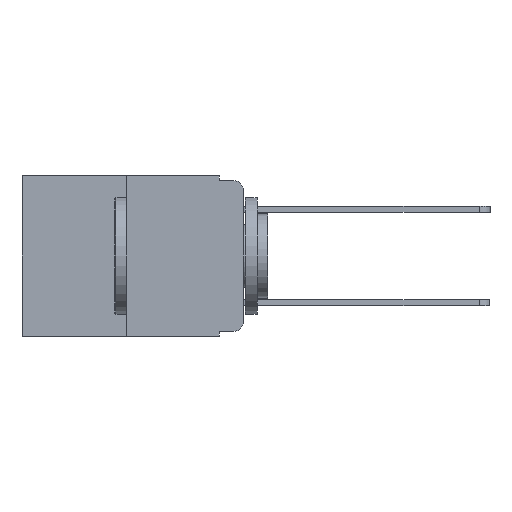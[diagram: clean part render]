
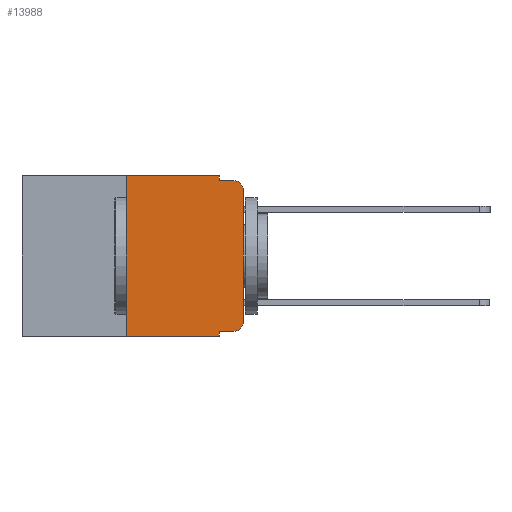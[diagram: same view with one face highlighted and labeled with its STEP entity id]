
A CAD part, left-side view. The second image highlights one B-rep face of the part: STEP entity #13988.
In plain terms, the highlighted planar face has unit normal (-1, 0, 0).
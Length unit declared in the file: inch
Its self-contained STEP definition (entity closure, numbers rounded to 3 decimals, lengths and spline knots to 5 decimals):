
#233 = EDGE_CURVE ( 'NONE', #7229, #4358, #17856, .T. ) ;
#365 = DIRECTION ( 'NONE',  ( 0., 0., 1. ) ) ;
#557 = LINE ( 'NONE', #856, #15821 ) ;
#856 = CARTESIAN_POINT ( 'NONE',  ( 0., 0.051, -0.01 ) ) ;
#885 = VECTOR ( 'NONE', #15459, 39.37008 ) ;
#1160 = VECTOR ( 'NONE', #2512, 39.37008 ) ;
#1750 = CARTESIAN_POINT ( 'NONE',  ( 0., 0.25, -0.343 ) ) ;
#2093 = ORIENTED_EDGE ( 'NONE', *, *, #9291, .F. ) ;
#2106 = ORIENTED_EDGE ( 'NONE', *, *, #10698, .F. ) ;
#2223 = CARTESIAN_POINT ( 'NONE',  ( 0., 0.02, -0.333 ) ) ;
#2512 = DIRECTION ( 'NONE',  ( 0., 0., 1. ) ) ;
#2616 = VERTEX_POINT ( 'NONE', #1750 ) ;
#2858 = ORIENTED_EDGE ( 'NONE', *, *, #9841, .T. ) ;
#3598 = LINE ( 'NONE', #12702, #11689 ) ;
#3950 = PLANE ( 'NONE',  #15090 ) ;
#4358 = VERTEX_POINT ( 'NONE', #13823 ) ;
#4474 = LINE ( 'NONE', #4968, #10679 ) ;
#4842 = ORIENTED_EDGE ( 'NONE', *, *, #16781, .T. ) ;
#4890 = CARTESIAN_POINT ( 'NONE',  ( 0., 0.051, 0. ) ) ;
#4935 = EDGE_LOOP ( 'NONE', ( #10047, #17041, #8863, #15759, #2093, #6054, #4842, #2106, #17639, #2858 ) ) ;
#4968 = CARTESIAN_POINT ( 'NONE',  ( 0., 0.473, 0. ) ) ;
#5125 = CARTESIAN_POINT ( 'NONE',  ( 0., 0.051, 0. ) ) ;
#5420 = LINE ( 'NONE', #16040, #1160 ) ;
#5471 = CARTESIAN_POINT ( 'NONE',  ( 0., 0.473, 0. ) ) ;
#5538 = DIRECTION ( 'NONE',  ( 0., 0., -1. ) ) ;
#5848 = DIRECTION ( 'NONE',  ( 0., -1., 0. ) ) ;
#6054 = ORIENTED_EDGE ( 'NONE', *, *, #18520, .F. ) ;
#6099 = CARTESIAN_POINT ( 'NONE',  ( 0., 0., -0.313 ) ) ;
#6383 = CARTESIAN_POINT ( 'NONE',  ( 0., 0., -0.03 ) ) ;
#7018 = LINE ( 'NONE', #9350, #14467 ) ;
#7178 = CARTESIAN_POINT ( 'NONE',  ( 0., 0.051, -0.333 ) ) ;
#7229 = VERTEX_POINT ( 'NONE', #6383 ) ;
#7263 = LINE ( 'NONE', #13284, #11710 ) ;
#7593 = CARTESIAN_POINT ( 'NONE',  ( 0., 0.051, 0. ) ) ;
#7651 = DIRECTION ( 'NONE',  ( -1., 0., 0. ) ) ;
#7738 = VERTEX_POINT ( 'NONE', #6099 ) ;
#8687 = DIRECTION ( 'NONE',  ( 0., -1., 0. ) ) ;
#8863 = ORIENTED_EDGE ( 'NONE', *, *, #17369, .F. ) ;
#9067 = EDGE_CURVE ( 'NONE', #14765, #12501, #11381, .T. ) ;
#9291 = EDGE_CURVE ( 'NONE', #16312, #14765, #4474, .T. ) ;
#9350 = CARTESIAN_POINT ( 'NONE',  ( 0., 0.051, -0.333 ) ) ;
#9841 = EDGE_CURVE ( 'NONE', #13312, #7738, #12709, .T. ) ;
#10000 = DIRECTION ( 'NONE',  ( 0., 0., -1. ) ) ;
#10047 = ORIENTED_EDGE ( 'NONE', *, *, #17182, .T. ) ;
#10455 = AXIS2_PLACEMENT_3D ( 'NONE', #16487, #7651, #17949 ) ;
#10679 = VECTOR ( 'NONE', #11018, 39.37008 ) ;
#10698 = EDGE_CURVE ( 'NONE', #18510, #12955, #16568, .T. ) ;
#11018 = DIRECTION ( 'NONE',  ( 0., -1., 0. ) ) ;
#11381 = LINE ( 'NONE', #4890, #18663 ) ;
#11689 = VECTOR ( 'NONE', #365, 39.37008 ) ;
#11710 = VECTOR ( 'NONE', #5848, 39.37008 ) ;
#12501 = VERTEX_POINT ( 'NONE', #18356 ) ;
#12702 = CARTESIAN_POINT ( 'NONE',  ( 0., 0., 0. ) ) ;
#12709 = CIRCLE ( 'NONE', #10455, 0.02 ) ;
#12955 = VERTEX_POINT ( 'NONE', #13490 ) ;
#13284 = CARTESIAN_POINT ( 'NONE',  ( 0., 0.473, -0.343 ) ) ;
#13312 = VERTEX_POINT ( 'NONE', #2223 ) ;
#13490 = CARTESIAN_POINT ( 'NONE',  ( 0., 0.051, -0.343 ) ) ;
#13823 = CARTESIAN_POINT ( 'NONE',  ( 0., 0.02, -0.01 ) ) ;
#13894 = DIRECTION ( 'NONE',  ( 0., 0., -1. ) ) ;
#13988 = ADVANCED_FACE ( 'NONE', ( #16850 ), #3950, .F. ) ;
#14467 = VECTOR ( 'NONE', #18129, 39.37008 ) ;
#14496 = DIRECTION ( 'NONE',  ( 1., 0., 0. ) ) ;
#14765 = VERTEX_POINT ( 'NONE', #7593 ) ;
#15090 = AXIS2_PLACEMENT_3D ( 'NONE', #5471, #14496, #5538 ) ;
#15177 = DIRECTION ( 'NONE',  ( -1., 0., 0. ) ) ;
#15459 = DIRECTION ( 'NONE',  ( 0., 0., -1. ) ) ;
#15759 = ORIENTED_EDGE ( 'NONE', *, *, #9067, .F. ) ;
#15821 = VECTOR ( 'NONE', #8687, 39.37008 ) ;
#16040 = CARTESIAN_POINT ( 'NONE',  ( 0., 0.25, 0. ) ) ;
#16312 = VERTEX_POINT ( 'NONE', #17966 ) ;
#16487 = CARTESIAN_POINT ( 'NONE',  ( 0., 0.02, -0.313 ) ) ;
#16568 = LINE ( 'NONE', #5125, #885 ) ;
#16781 = EDGE_CURVE ( 'NONE', #2616, #12955, #7263, .T. ) ;
#16850 = FACE_OUTER_BOUND ( 'NONE', #4935, .T. ) ;
#16973 = AXIS2_PLACEMENT_3D ( 'NONE', #17811, #15177, #10000 ) ;
#17025 = EDGE_CURVE ( 'NONE', #18510, #13312, #7018, .T. ) ;
#17041 = ORIENTED_EDGE ( 'NONE', *, *, #233, .T. ) ;
#17182 = EDGE_CURVE ( 'NONE', #7738, #7229, #3598, .T. ) ;
#17369 = EDGE_CURVE ( 'NONE', #12501, #4358, #557, .T. ) ;
#17639 = ORIENTED_EDGE ( 'NONE', *, *, #17025, .T. ) ;
#17811 = CARTESIAN_POINT ( 'NONE',  ( 0., 0.02, -0.03 ) ) ;
#17856 = CIRCLE ( 'NONE', #16973, 0.02 ) ;
#17949 = DIRECTION ( 'NONE',  ( 0., 0., -1. ) ) ;
#17966 = CARTESIAN_POINT ( 'NONE',  ( 0., 0.25, 0. ) ) ;
#18129 = DIRECTION ( 'NONE',  ( 0., -1., 0. ) ) ;
#18356 = CARTESIAN_POINT ( 'NONE',  ( 0., 0.051, -0.01 ) ) ;
#18510 = VERTEX_POINT ( 'NONE', #7178 ) ;
#18520 = EDGE_CURVE ( 'NONE', #2616, #16312, #5420, .T. ) ;
#18663 = VECTOR ( 'NONE', #13894, 39.37008 ) ;
